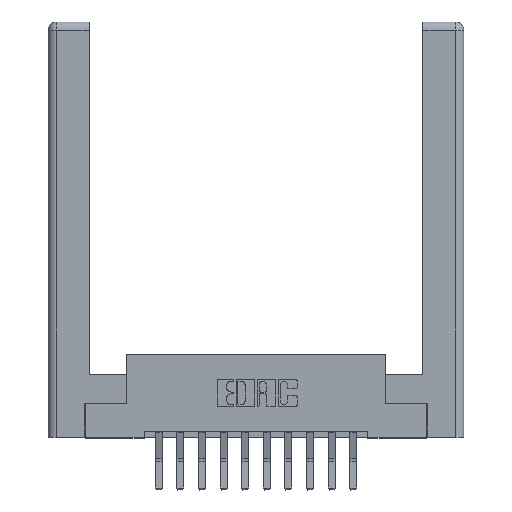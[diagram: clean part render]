
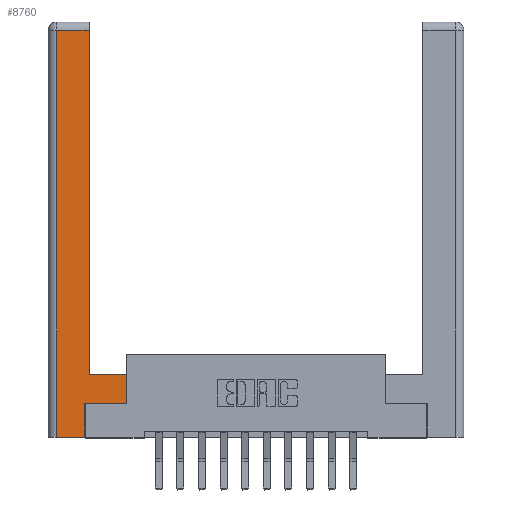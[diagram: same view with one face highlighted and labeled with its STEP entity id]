
A CAD part, top view. The second image highlights one B-rep face of the part: STEP entity #8760.
In plain terms, the highlighted planar face has unit normal (0, 0, 1).
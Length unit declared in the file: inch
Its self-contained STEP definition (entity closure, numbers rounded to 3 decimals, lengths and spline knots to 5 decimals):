
#78 = CARTESIAN_POINT ( 'NONE',  ( 0.565, 0.45, 0. ) ) ;
#553 = ORIENTED_EDGE ( 'NONE', *, *, #10509, .T. ) ;
#1108 = CARTESIAN_POINT ( 'NONE',  ( 0.265, 0., 0. ) ) ;
#1420 = DIRECTION ( 'NONE',  ( 0., 1., 0. ) ) ;
#1457 = CARTESIAN_POINT ( 'NONE',  ( 0.295, 0.45, 0. ) ) ;
#1660 = DIRECTION ( 'NONE',  ( 1., 0., 0. ) ) ;
#1714 = LINE ( 'NONE', #10348, #11596 ) ;
#1823 = EDGE_CURVE ( 'NONE', #9737, #3369, #5821, .T. ) ;
#1881 = LINE ( 'NONE', #2035, #3824 ) ;
#2035 = CARTESIAN_POINT ( 'NONE',  ( 0.295, 3., 0. ) ) ;
#2085 = DIRECTION ( 'NONE',  ( -1., 0., 0. ) ) ;
#2310 = VECTOR ( 'NONE', #1420, 39.37008 ) ;
#2545 = ORIENTED_EDGE ( 'NONE', *, *, #14220, .T. ) ;
#2846 = DIRECTION ( 'NONE',  ( 0., 1., 0. ) ) ;
#3368 = DIRECTION ( 'NONE',  ( -1., 0., 0. ) ) ;
#3369 = VERTEX_POINT ( 'NONE', #13630 ) ;
#3660 = VERTEX_POINT ( 'NONE', #3788 ) ;
#3717 = EDGE_CURVE ( 'NONE', #8748, #4669, #13086, .T. ) ;
#3788 = CARTESIAN_POINT ( 'NONE',  ( 0.565, 0.245, 0. ) ) ;
#3799 = PLANE ( 'NONE',  #8390 ) ;
#3824 = VECTOR ( 'NONE', #5497, 39.37008 ) ;
#3903 = CARTESIAN_POINT ( 'NONE',  ( 0.265, 0.245, 0. ) ) ;
#3936 = CARTESIAN_POINT ( 'NONE',  ( 0., 0., 0. ) ) ;
#4310 = VERTEX_POINT ( 'NONE', #1457 ) ;
#4669 = VERTEX_POINT ( 'NONE', #3903 ) ;
#5216 = CARTESIAN_POINT ( 'NONE',  ( 0.265, 0.245, 0. ) ) ;
#5293 = LINE ( 'NONE', #78, #2310 ) ;
#5497 = DIRECTION ( 'NONE',  ( 0., 1., 0. ) ) ;
#5821 = LINE ( 'NONE', #12179, #11446 ) ;
#5868 = EDGE_CURVE ( 'NONE', #11740, #4310, #8946, .T. ) ;
#5972 = VERTEX_POINT ( 'NONE', #6053 ) ;
#6053 = CARTESIAN_POINT ( 'NONE',  ( 0.0615, 0., 0. ) ) ;
#6581 = FACE_OUTER_BOUND ( 'NONE', #14221, .T. ) ;
#6895 = EDGE_CURVE ( 'NONE', #4310, #9737, #1881, .T. ) ;
#7016 = ORIENTED_EDGE ( 'NONE', *, *, #3717, .T. ) ;
#7039 = VECTOR ( 'NONE', #3368, 39.37008 ) ;
#7462 = EDGE_CURVE ( 'NONE', #5972, #8748, #12630, .T. ) ;
#8263 = DIRECTION ( 'NONE',  ( -1., 0., 0. ) ) ;
#8288 = ORIENTED_EDGE ( 'NONE', *, *, #5868, .T. ) ;
#8309 = CARTESIAN_POINT ( 'NONE',  ( 0.265, 0., 0. ) ) ;
#8390 = AXIS2_PLACEMENT_3D ( 'NONE', #3936, #11811, #8263 ) ;
#8748 = VERTEX_POINT ( 'NONE', #8309 ) ;
#8760 = ADVANCED_FACE ( 'NONE', ( #6581 ), #3799, .F. ) ;
#8802 = ORIENTED_EDGE ( 'NONE', *, *, #1823, .T. ) ;
#8851 = DIRECTION ( 'NONE',  ( 1., 0., 0. ) ) ;
#8946 = LINE ( 'NONE', #10091, #7039 ) ;
#9687 = EDGE_CURVE ( 'NONE', #3660, #11740, #5293, .T. ) ;
#9737 = VERTEX_POINT ( 'NONE', #11477 ) ;
#9843 = DIRECTION ( 'NONE',  ( 0., -1., 0. ) ) ;
#10091 = CARTESIAN_POINT ( 'NONE',  ( 0.295, 0.45, 0. ) ) ;
#10348 = CARTESIAN_POINT ( 'NONE',  ( 0.0615, 0., 0. ) ) ;
#10452 = LINE ( 'NONE', #14293, #12038 ) ;
#10509 = EDGE_CURVE ( 'NONE', #3369, #5972, #1714, .T. ) ;
#10588 = VECTOR ( 'NONE', #2846, 39.37008 ) ;
#11397 = VECTOR ( 'NONE', #8851, 39.37008 ) ;
#11446 = VECTOR ( 'NONE', #2085, 39.37008 ) ;
#11477 = CARTESIAN_POINT ( 'NONE',  ( 0.295, 2.94, 0. ) ) ;
#11596 = VECTOR ( 'NONE', #9843, 39.37008 ) ;
#11740 = VERTEX_POINT ( 'NONE', #12593 ) ;
#11811 = DIRECTION ( 'NONE',  ( 0., 0., -1. ) ) ;
#12038 = VECTOR ( 'NONE', #1660, 39.37008 ) ;
#12179 = CARTESIAN_POINT ( 'NONE',  ( 0.0615, 2.94, 0. ) ) ;
#12323 = ORIENTED_EDGE ( 'NONE', *, *, #7462, .T. ) ;
#12593 = CARTESIAN_POINT ( 'NONE',  ( 0.565, 0.45, 0. ) ) ;
#12630 = LINE ( 'NONE', #1108, #11397 ) ;
#12804 = ORIENTED_EDGE ( 'NONE', *, *, #6895, .T. ) ;
#13086 = LINE ( 'NONE', #5216, #10588 ) ;
#13630 = CARTESIAN_POINT ( 'NONE',  ( 0.0615, 2.94, 0. ) ) ;
#13931 = ORIENTED_EDGE ( 'NONE', *, *, #9687, .T. ) ;
#14220 = EDGE_CURVE ( 'NONE', #4669, #3660, #10452, .T. ) ;
#14221 = EDGE_LOOP ( 'NONE', ( #12804, #8802, #553, #12323, #7016, #2545, #13931, #8288 ) ) ;
#14293 = CARTESIAN_POINT ( 'NONE',  ( 0.565, 0.245, 0. ) ) ;
